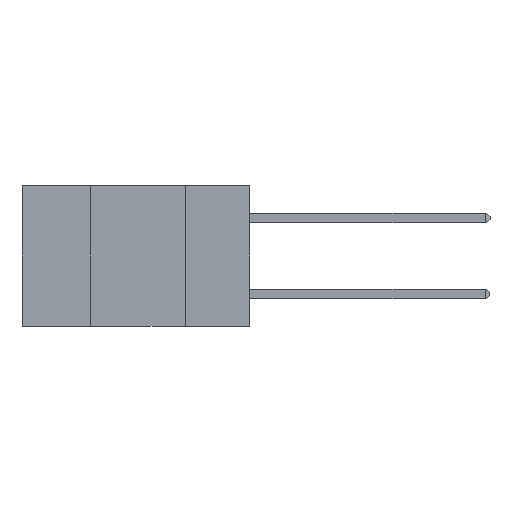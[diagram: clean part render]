
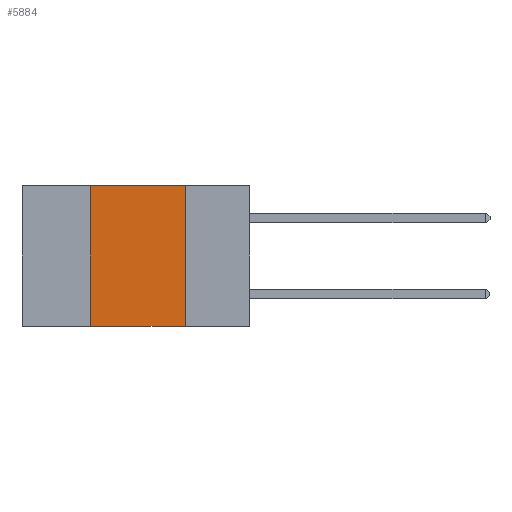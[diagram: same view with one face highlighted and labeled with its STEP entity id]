
A CAD part, left-side view. The second image highlights one B-rep face of the part: STEP entity #5884.
In plain terms, the highlighted planar face has unit normal (-1, 0, 0).
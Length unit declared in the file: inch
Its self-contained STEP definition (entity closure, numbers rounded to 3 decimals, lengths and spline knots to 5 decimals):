
#615 = ORIENTED_EDGE ( 'NONE', *, *, #14750, .F. ) ;
#1085 = CARTESIAN_POINT ( 'NONE',  ( 0., 0.6, 0. ) ) ;
#1090 = DIRECTION ( 'NONE',  ( 0., -1., 0. ) ) ;
#1150 = DIRECTION ( 'NONE',  ( 0., 0., 1. ) ) ;
#1625 = DIRECTION ( 'NONE',  ( 0., 0., -1. ) ) ;
#2119 = LINE ( 'NONE', #12738, #4935 ) ;
#2878 = EDGE_CURVE ( 'NONE', #10439, #8163, #3941, .T. ) ;
#3395 = LINE ( 'NONE', #11824, #12527 ) ;
#3484 = FACE_OUTER_BOUND ( 'NONE', #10240, .T. ) ;
#3815 = ORIENTED_EDGE ( 'NONE', *, *, #7694, .T. ) ;
#3941 = LINE ( 'NONE', #7610, #6793 ) ;
#4511 = DIRECTION ( 'NONE',  ( 0., -1., 0. ) ) ;
#4749 = VERTEX_POINT ( 'NONE', #7395 ) ;
#4763 = PLANE ( 'NONE',  #11153 ) ;
#4935 = VECTOR ( 'NONE', #4511, 39.37008 ) ;
#4970 = CARTESIAN_POINT ( 'NONE',  ( 0., 0.17, 0. ) ) ;
#5099 = ORIENTED_EDGE ( 'NONE', *, *, #7555, .F. ) ;
#5884 = ADVANCED_FACE ( 'NONE', ( #3484 ), #4763, .F. ) ;
#5971 = DIRECTION ( 'NONE',  ( 0., 0., -1. ) ) ;
#6266 = VECTOR ( 'NONE', #1150, 39.37008 ) ;
#6700 = ORIENTED_EDGE ( 'NONE', *, *, #2878, .F. ) ;
#6793 = VECTOR ( 'NONE', #1625, 39.37008 ) ;
#7395 = CARTESIAN_POINT ( 'NONE',  ( 0., 0.42, -0.37 ) ) ;
#7555 = EDGE_CURVE ( 'NONE', #7861, #10439, #2119, .T. ) ;
#7610 = CARTESIAN_POINT ( 'NONE',  ( 0., 0.17, 0. ) ) ;
#7694 = EDGE_CURVE ( 'NONE', #4749, #8163, #3395, .T. ) ;
#7861 = VERTEX_POINT ( 'NONE', #14441 ) ;
#8163 = VERTEX_POINT ( 'NONE', #10360 ) ;
#9058 = LINE ( 'NONE', #9593, #6266 ) ;
#9593 = CARTESIAN_POINT ( 'NONE',  ( 0., 0.42, 0. ) ) ;
#10240 = EDGE_LOOP ( 'NONE', ( #6700, #5099, #615, #3815 ) ) ;
#10360 = CARTESIAN_POINT ( 'NONE',  ( 0., 0.17, -0.37 ) ) ;
#10439 = VERTEX_POINT ( 'NONE', #4970 ) ;
#11153 = AXIS2_PLACEMENT_3D ( 'NONE', #1085, #13038, #5971 ) ;
#11824 = CARTESIAN_POINT ( 'NONE',  ( 0., 0.6, -0.37 ) ) ;
#12527 = VECTOR ( 'NONE', #1090, 39.37008 ) ;
#12738 = CARTESIAN_POINT ( 'NONE',  ( 0., 0.6, 0. ) ) ;
#13038 = DIRECTION ( 'NONE',  ( 1., 0., 0. ) ) ;
#14441 = CARTESIAN_POINT ( 'NONE',  ( 0., 0.42, 0. ) ) ;
#14750 = EDGE_CURVE ( 'NONE', #4749, #7861, #9058, .T. ) ;
